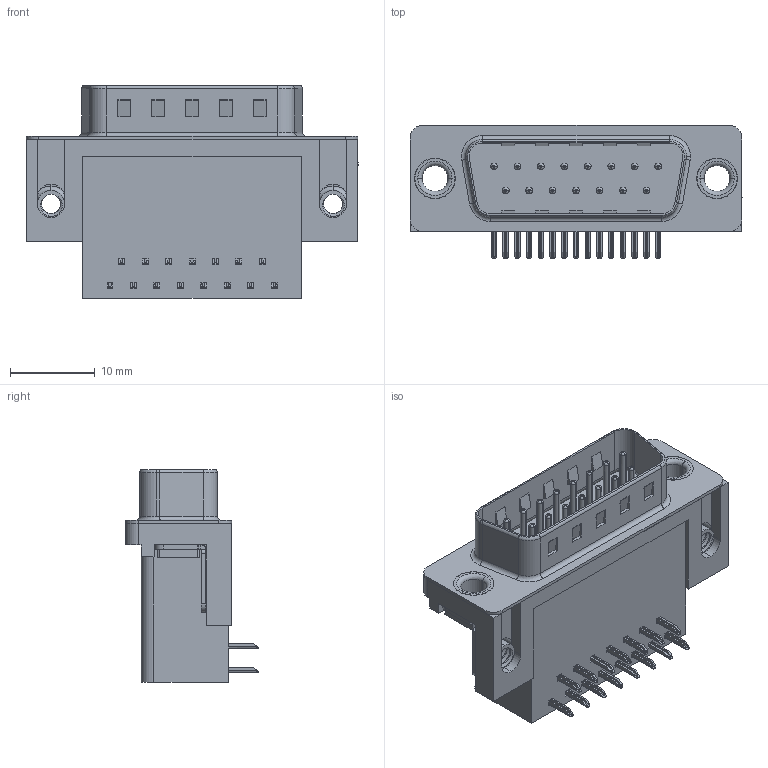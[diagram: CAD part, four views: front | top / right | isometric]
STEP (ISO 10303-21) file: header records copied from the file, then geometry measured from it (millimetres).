
FILE_DESCRIPTION (( 'STEP AP203' ), '1' );
FILE_NAME ('625-015-362-051.STEP', '2018-11-05T23:33:20', ( '' ), ( '' ), 'SwSTEP 2.0', 'SolidWorks 2016', '' );
FILE_SCHEMA (( 'CONFIG_CONTROL_DESIGN' ));
Length unit declared in the file: millimetre
Products named in the file (7): 625-015-362-051; 625 Housing_15 Socket; 625 Shell_15 Socket; 625 Contact Bottom; 625 Contact Top; 625 4-40 Threaded Board Mount; 625 Thru Hole Rivet
Assembly tree (21 placements, depth 2):
  625-015-362-051
    625 Housing_15 Socket
    625 Shell_15 Socket
    625 Contact Bottom  x7
    625 Contact Top  x8
    625 4-40 Threaded Board Mount  x2
    625 Thru Hole Rivet  x2
Bounding box: 39.22 x 15.73 x 25.16 mm (x, y, z)
Volume: 6241.6 mm3; surface area: 6480.5 mm2
Topology: 21 solids, 21 shells, 1471 faces, 3657 edges, 2267 vertices
Faces by surface type: plane 895, cylinder 441, torus 129, bspline 6
Entity records: 18595 total; most frequent: CARTESIAN_POINT 4242, DIRECTION 2821, ORIENTED_EDGE 2692, EDGE_CURVE 1346, AXIS2_PLACEMENT_3D 953, LINE 915, VECTOR 915, VERTEX_POINT 859
